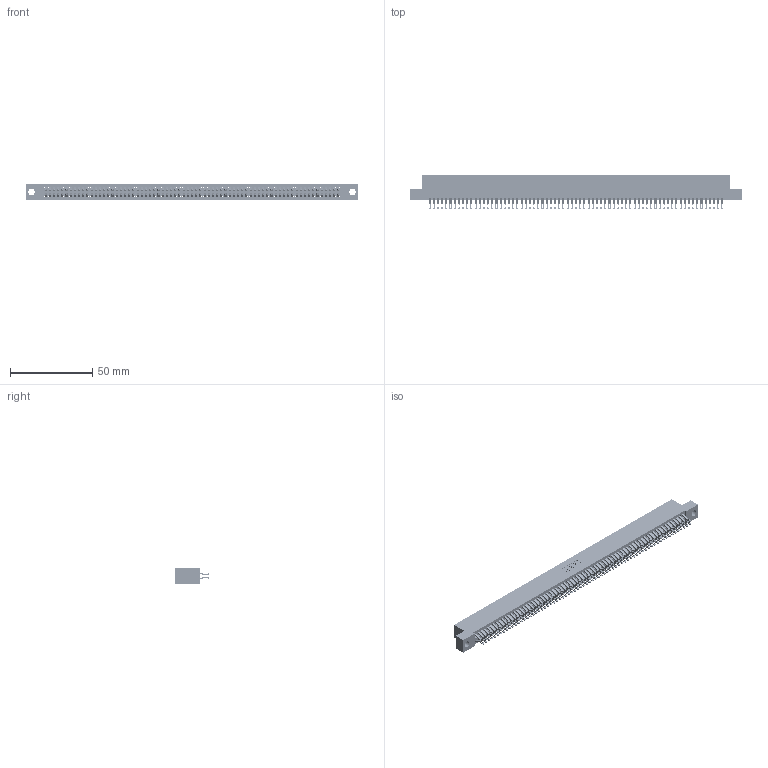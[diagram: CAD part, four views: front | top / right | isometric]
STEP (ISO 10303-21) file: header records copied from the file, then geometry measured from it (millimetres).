
FILE_DESCRIPTION (( 'STEP AP203' ), '1' );
FILE_NAME ('395-142-555-204.STEP', '2021-06-18T05:35:49', ( '' ), ( '' ), 'SwSTEP 2.0', 'SolidWorks 2020', '' );
FILE_SCHEMA (( 'CONFIG_CONTROL_DESIGN' ));
Length unit declared in the file: inch
Products named in the file (3): 345 Part_Flush Mounting Lugs - 0.156 Dia-TI; 345-292-001_555 Tail; 395-142-555-204
Assembly tree (143 placements, depth 2):
  395-142-555-204
    345 Part_Flush Mounting Lugs - 0.156 Dia-TI
    345-292-001_555 Tail  x142
Bounding box: 201.55 x 21.13 x 9.4 mm (x, y, z)
Volume: 20153.8 mm3; surface area: 31636.5 mm2
Topology: 143 solids, 143 shells, 8092 faces, 25511 edges, 17006 vertices
Faces by surface type: plane 4496, cylinder 3596
Entity records: 52549 total; most frequent: CARTESIAN_POINT 8820, ORIENTED_EDGE 8722, DIRECTION 7709, EDGE_CURVE 4361, VECTOR 3925, LINE 3925, VERTEX_POINT 2906, AXIS2_PLACEMENT_3D 1892
